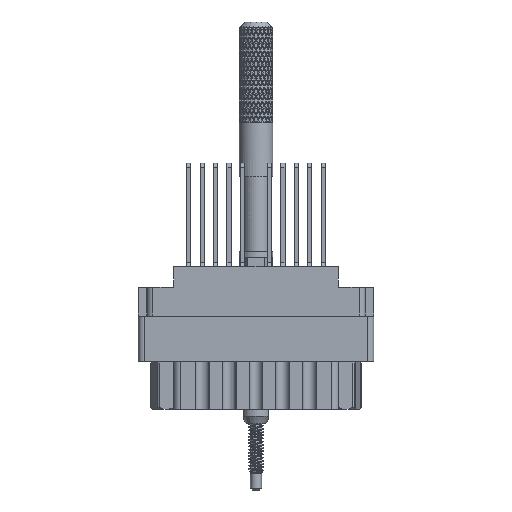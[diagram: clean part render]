
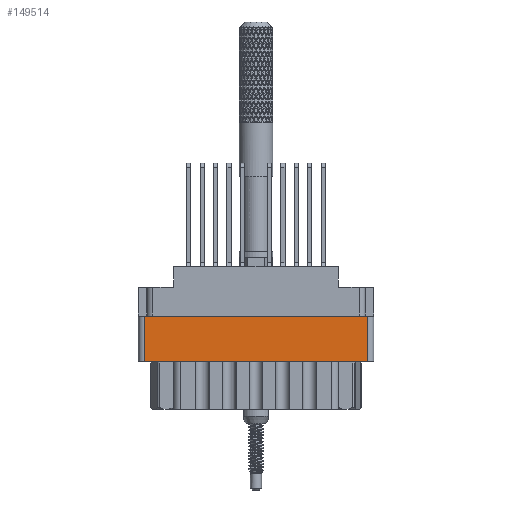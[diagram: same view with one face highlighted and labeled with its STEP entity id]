
A CAD part, front view. The second image highlights one B-rep face of the part: STEP entity #149514.
In plain terms, the highlighted planar face has unit normal (0, -1, 0).
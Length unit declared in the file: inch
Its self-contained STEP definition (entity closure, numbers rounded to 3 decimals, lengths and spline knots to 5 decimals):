
#3098 = VECTOR ( 'NONE', #10525, 39.37008 ) ;
#3346 = ORIENTED_EDGE ( 'NONE', *, *, #43574, .T. ) ;
#10525 = DIRECTION ( 'NONE',  ( 1., 0., 0. ) ) ;
#13307 = LINE ( 'NONE', #91240, #176981 ) ;
#23202 = EDGE_CURVE ( 'NONE', #177706, #144961, #13307, .T. ) ;
#25451 = PLANE ( 'NONE',  #50910 ) ;
#26129 = CARTESIAN_POINT ( 'NONE',  ( 0.624, -0.343, -0.277 ) ) ;
#27435 = VERTEX_POINT ( 'NONE', #45205 ) ;
#29666 = DIRECTION ( 'NONE',  ( 0., 0., 1. ) ) ;
#36603 = CARTESIAN_POINT ( 'NONE',  ( -0.624, -0.343, -0.798 ) ) ;
#40687 = DIRECTION ( 'NONE',  ( 0., 0., -1. ) ) ;
#43574 = EDGE_CURVE ( 'NONE', #27435, #77938, #141949, .T. ) ;
#44826 = ORIENTED_EDGE ( 'NONE', *, *, #116141, .F. ) ;
#45205 = CARTESIAN_POINT ( 'NONE',  ( -0.624, -0.343, -0.277 ) ) ;
#47633 = ORIENTED_EDGE ( 'NONE', *, *, #23202, .T. ) ;
#47736 = CARTESIAN_POINT ( 'NONE',  ( -0.624, -0.343, -0.529 ) ) ;
#48158 = LINE ( 'NONE', #84740, #3098 ) ;
#50910 = AXIS2_PLACEMENT_3D ( 'NONE', #70509, #132143, #40687 ) ;
#68265 = VECTOR ( 'NONE', #162141, 39.37008 ) ;
#70509 = CARTESIAN_POINT ( 'NONE',  ( -0.656, -0.343, -0.798 ) ) ;
#77938 = VERTEX_POINT ( 'NONE', #47736 ) ;
#84740 = CARTESIAN_POINT ( 'NONE',  ( 0., -0.343, -0.277 ) ) ;
#87225 = LINE ( 'NONE', #101208, #68265 ) ;
#91240 = CARTESIAN_POINT ( 'NONE',  ( 0.624, -0.343, -0.798 ) ) ;
#93788 = EDGE_CURVE ( 'NONE', #177706, #77938, #87225, .T. ) ;
#95044 = DIRECTION ( 'NONE',  ( 0., 0., -1. ) ) ;
#101208 = CARTESIAN_POINT ( 'NONE',  ( 0., -0.343, -0.529 ) ) ;
#114347 = FACE_OUTER_BOUND ( 'NONE', #117680, .T. ) ;
#116141 = EDGE_CURVE ( 'NONE', #27435, #144961, #48158, .T. ) ;
#117680 = EDGE_LOOP ( 'NONE', ( #44826, #3346, #154782, #47633 ) ) ;
#130132 = VECTOR ( 'NONE', #95044, 39.37008 ) ;
#132143 = DIRECTION ( 'NONE',  ( 0., -1., 0. ) ) ;
#141949 = LINE ( 'NONE', #36603, #130132 ) ;
#144961 = VERTEX_POINT ( 'NONE', #26129 ) ;
#149514 = ADVANCED_FACE ( 'NONE', ( #114347 ), #25451, .T. ) ;
#154782 = ORIENTED_EDGE ( 'NONE', *, *, #93788, .F. ) ;
#162141 = DIRECTION ( 'NONE',  ( -1., 0., 0. ) ) ;
#171163 = CARTESIAN_POINT ( 'NONE',  ( 0.624, -0.343, -0.529 ) ) ;
#176981 = VECTOR ( 'NONE', #29666, 39.37008 ) ;
#177706 = VERTEX_POINT ( 'NONE', #171163 ) ;
